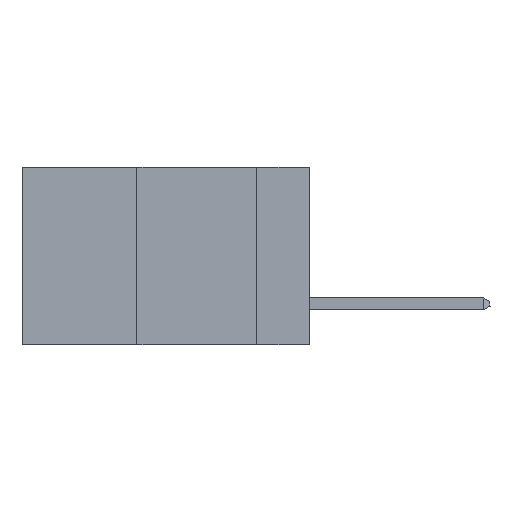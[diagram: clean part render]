
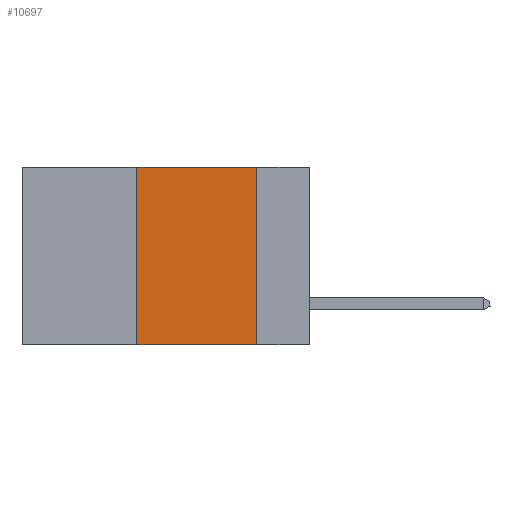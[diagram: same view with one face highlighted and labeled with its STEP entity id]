
A CAD part, left-side view. The second image highlights one B-rep face of the part: STEP entity #10697.
In plain terms, the highlighted planar face has unit normal (-1, 0, 0).
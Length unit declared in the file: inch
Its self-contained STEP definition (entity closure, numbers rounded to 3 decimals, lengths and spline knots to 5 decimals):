
#932 = CARTESIAN_POINT ( 'NONE',  ( 0., 0.11, -0.37 ) ) ;
#2499 = FACE_OUTER_BOUND ( 'NONE', #19166, .T. ) ;
#3862 = EDGE_CURVE ( 'NONE', #32791, #20252, #32317, .T. ) ;
#4121 = ORIENTED_EDGE ( 'NONE', *, *, #32672, .F. ) ;
#4831 = VERTEX_POINT ( 'NONE', #932 ) ;
#5943 = DIRECTION ( 'NONE',  ( 0., 0., -1. ) ) ;
#6535 = VECTOR ( 'NONE', #27722, 39.37008 ) ;
#7805 = ORIENTED_EDGE ( 'NONE', *, *, #3862, .F. ) ;
#8919 = LINE ( 'NONE', #18862, #20296 ) ;
#9479 = DIRECTION ( 'NONE',  ( 0., -1., 0. ) ) ;
#10697 = ADVANCED_FACE ( 'NONE', ( #2499 ), #11108, .F. ) ;
#10774 = CARTESIAN_POINT ( 'NONE',  ( 0., 0.36, 0. ) ) ;
#11108 = PLANE ( 'NONE',  #35974 ) ;
#12917 = LINE ( 'NONE', #10774, #35223 ) ;
#15932 = LINE ( 'NONE', #21969, #22817 ) ;
#17120 = ORIENTED_EDGE ( 'NONE', *, *, #34967, .F. ) ;
#17867 = DIRECTION ( 'NONE',  ( 1., 0., 0. ) ) ;
#18862 = CARTESIAN_POINT ( 'NONE',  ( 0., 0.6, -0.37 ) ) ;
#19166 = EDGE_LOOP ( 'NONE', ( #17120, #7805, #4121, #25096 ) ) ;
#20252 = VERTEX_POINT ( 'NONE', #35143 ) ;
#20296 = VECTOR ( 'NONE', #9479, 39.37008 ) ;
#21969 = CARTESIAN_POINT ( 'NONE',  ( 0., 0.11, 0. ) ) ;
#22817 = VECTOR ( 'NONE', #5943, 39.37008 ) ;
#25096 = ORIENTED_EDGE ( 'NONE', *, *, #36061, .T. ) ;
#26930 = CARTESIAN_POINT ( 'NONE',  ( 0., 0.36, 0. ) ) ;
#27133 = CARTESIAN_POINT ( 'NONE',  ( 0., 0.6, 0. ) ) ;
#27722 = DIRECTION ( 'NONE',  ( 0., -1., 0. ) ) ;
#32204 = CARTESIAN_POINT ( 'NONE',  ( 0., 0.36, -0.37 ) ) ;
#32317 = LINE ( 'NONE', #40414, #6535 ) ;
#32672 = EDGE_CURVE ( 'NONE', #33839, #32791, #12917, .T. ) ;
#32791 = VERTEX_POINT ( 'NONE', #26930 ) ;
#33058 = DIRECTION ( 'NONE',  ( 0., 0., 1. ) ) ;
#33839 = VERTEX_POINT ( 'NONE', #32204 ) ;
#34967 = EDGE_CURVE ( 'NONE', #20252, #4831, #15932, .T. ) ;
#35143 = CARTESIAN_POINT ( 'NONE',  ( 0., 0.11, 0. ) ) ;
#35223 = VECTOR ( 'NONE', #33058, 39.37008 ) ;
#35974 = AXIS2_PLACEMENT_3D ( 'NONE', #27133, #17867, #39587 ) ;
#36061 = EDGE_CURVE ( 'NONE', #33839, #4831, #8919, .T. ) ;
#39587 = DIRECTION ( 'NONE',  ( 0., 0., -1. ) ) ;
#40414 = CARTESIAN_POINT ( 'NONE',  ( 0., 0.6, 0. ) ) ;
